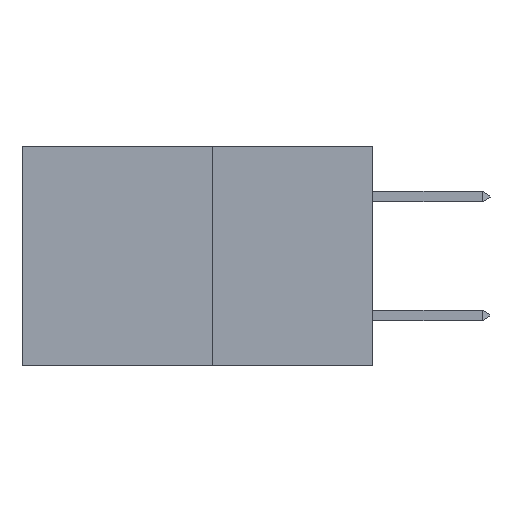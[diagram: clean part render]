
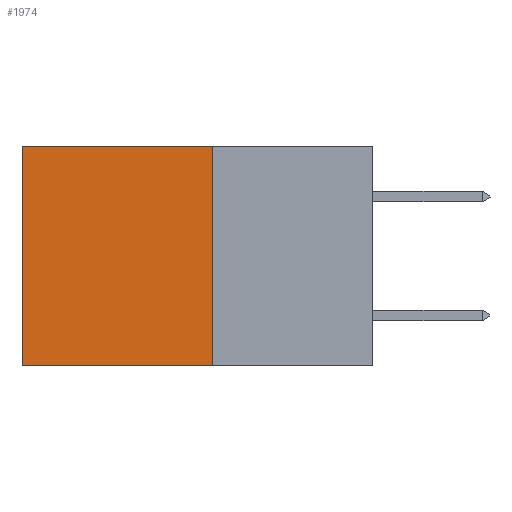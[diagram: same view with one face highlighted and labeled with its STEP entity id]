
A CAD part, left-side view. The second image highlights one B-rep face of the part: STEP entity #1974.
In plain terms, the highlighted planar face has unit normal (-1, 0, 0).
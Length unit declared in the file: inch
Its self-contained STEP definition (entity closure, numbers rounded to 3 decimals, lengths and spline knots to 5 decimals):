
#197 = CARTESIAN_POINT ( 'NONE',  ( 0.277, 0.27, 0. ) ) ;
#306 = ORIENTED_EDGE ( 'NONE', *, *, #13459, .T. ) ;
#327 = VECTOR ( 'NONE', #2392, 39.37008 ) ;
#945 = VERTEX_POINT ( 'NONE', #7348 ) ;
#1202 = LINE ( 'NONE', #12702, #4294 ) ;
#1546 = EDGE_CURVE ( 'NONE', #13429, #9754, #15747, .T. ) ;
#1974 = ADVANCED_FACE ( 'NONE', ( #8969 ), #8657, .F. ) ;
#2019 = DIRECTION ( 'NONE',  ( 0., 0., -1. ) ) ;
#2392 = DIRECTION ( 'NONE',  ( 0., 1., 0. ) ) ;
#2765 = ORIENTED_EDGE ( 'NONE', *, *, #3499, .T. ) ;
#2965 = ORIENTED_EDGE ( 'NONE', *, *, #4328, .F. ) ;
#3499 = EDGE_CURVE ( 'NONE', #12242, #9754, #1202, .T. ) ;
#3710 = CARTESIAN_POINT ( 'NONE',  ( 0.277, 0.59, -0.37 ) ) ;
#4294 = VECTOR ( 'NONE', #2019, 39.37008 ) ;
#4328 = EDGE_CURVE ( 'NONE', #945, #13429, #5918, .T. ) ;
#4686 = DIRECTION ( 'NONE',  ( 0., 0., -1. ) ) ;
#4779 = CARTESIAN_POINT ( 'NONE',  ( 0.277, 0.27, -0.37 ) ) ;
#5918 = LINE ( 'NONE', #15906, #9262 ) ;
#7348 = CARTESIAN_POINT ( 'NONE',  ( 0.277, 0.27, 0. ) ) ;
#8657 = PLANE ( 'NONE',  #10464 ) ;
#8748 = CARTESIAN_POINT ( 'NONE',  ( 0.277, 0.59, 0. ) ) ;
#8969 = FACE_OUTER_BOUND ( 'NONE', #12940, .T. ) ;
#9262 = VECTOR ( 'NONE', #4686, 39.37008 ) ;
#9754 = VERTEX_POINT ( 'NONE', #3710 ) ;
#10464 = AXIS2_PLACEMENT_3D ( 'NONE', #14266, #15666, #11310 ) ;
#11310 = DIRECTION ( 'NONE',  ( 0., 0., -1. ) ) ;
#11741 = ORIENTED_EDGE ( 'NONE', *, *, #1546, .F. ) ;
#12242 = VERTEX_POINT ( 'NONE', #8748 ) ;
#12702 = CARTESIAN_POINT ( 'NONE',  ( 0.277, 0.59, -0.37 ) ) ;
#12940 = EDGE_LOOP ( 'NONE', ( #2765, #11741, #2965, #306 ) ) ;
#13429 = VERTEX_POINT ( 'NONE', #4779 ) ;
#13459 = EDGE_CURVE ( 'NONE', #945, #12242, #13793, .T. ) ;
#13793 = LINE ( 'NONE', #197, #327 ) ;
#14266 = CARTESIAN_POINT ( 'NONE',  ( 0.277, 0.27, -0.37 ) ) ;
#14569 = CARTESIAN_POINT ( 'NONE',  ( 0.277, 0.27, -0.37 ) ) ;
#14993 = DIRECTION ( 'NONE',  ( 0., 1., 0. ) ) ;
#15011 = VECTOR ( 'NONE', #14993, 39.37008 ) ;
#15666 = DIRECTION ( 'NONE',  ( 1., 0., 0. ) ) ;
#15747 = LINE ( 'NONE', #14569, #15011 ) ;
#15906 = CARTESIAN_POINT ( 'NONE',  ( 0.277, 0.27, -0.37 ) ) ;
